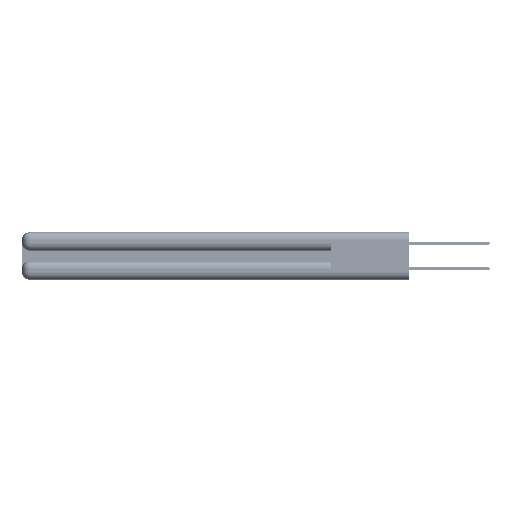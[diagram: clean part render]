
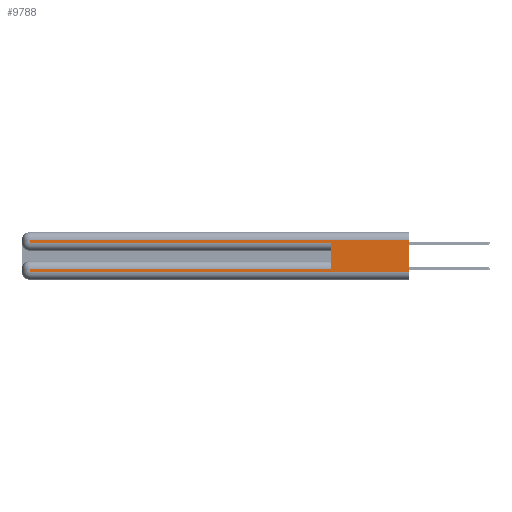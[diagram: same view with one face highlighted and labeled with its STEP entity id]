
A CAD part, left-side view. The second image highlights one B-rep face of the part: STEP entity #9788.
In plain terms, the highlighted planar face has unit normal (-1, 0, 0).
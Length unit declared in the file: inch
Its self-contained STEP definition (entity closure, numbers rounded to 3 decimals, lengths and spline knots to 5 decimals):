
#1102 = VECTOR ( 'NONE', #44371, 39.37008 ) ;
#1187 = CARTESIAN_POINT ( 'NONE',  ( 0., 0., 0.285 ) ) ;
#2878 = CARTESIAN_POINT ( 'NONE',  ( 0., 2.94, 0.285 ) ) ;
#3086 = CARTESIAN_POINT ( 'NONE',  ( 0., 0., 0.37 ) ) ;
#3756 = CARTESIAN_POINT ( 'NONE',  ( 0., 0., 0.06 ) ) ;
#4195 = CARTESIAN_POINT ( 'NONE',  ( 0., 2.94, 0.085 ) ) ;
#4802 = CARTESIAN_POINT ( 'NONE',  ( 0., 0., 0.37 ) ) ;
#5175 = DIRECTION ( 'NONE',  ( 0., 0., -1. ) ) ;
#5289 = EDGE_CURVE ( 'NONE', #52848, #55226, #8378, .T. ) ;
#5853 = LINE ( 'NONE', #35079, #46763 ) ;
#6275 = DIRECTION ( 'NONE',  ( 0., -1., 0. ) ) ;
#7104 = DIRECTION ( 'NONE',  ( 0., 0., -1. ) ) ;
#7128 = VECTOR ( 'NONE', #55482, 39.37008 ) ;
#8378 = LINE ( 'NONE', #32959, #16560 ) ;
#8469 = VERTEX_POINT ( 'NONE', #21962 ) ;
#8534 = ORIENTED_EDGE ( 'NONE', *, *, #32265, .T. ) ;
#9788 = ADVANCED_FACE ( 'NONE', ( #42349 ), #50697, .F. ) ;
#11920 = AXIS2_PLACEMENT_3D ( 'NONE', #3086, #24656, #7104 ) ;
#12340 = EDGE_CURVE ( 'NONE', #14907, #27294, #5853, .T. ) ;
#12883 = ORIENTED_EDGE ( 'NONE', *, *, #45761, .F. ) ;
#14907 = VERTEX_POINT ( 'NONE', #55323 ) ;
#15025 = DIRECTION ( 'NONE',  ( 0., 0., 1. ) ) ;
#16560 = VECTOR ( 'NONE', #36776, 39.37008 ) ;
#18267 = ORIENTED_EDGE ( 'NONE', *, *, #26750, .T. ) ;
#18658 = ORIENTED_EDGE ( 'NONE', *, *, #43704, .T. ) ;
#19375 = CARTESIAN_POINT ( 'NONE',  ( 0., 0., 0.31 ) ) ;
#20033 = CARTESIAN_POINT ( 'NONE',  ( 0., 0.6, 0.085 ) ) ;
#20605 = LINE ( 'NONE', #1187, #53283 ) ;
#21962 = CARTESIAN_POINT ( 'NONE',  ( 0., 0., 0.06 ) ) ;
#23634 = CARTESIAN_POINT ( 'NONE',  ( 0., 0.6, 0.145 ) ) ;
#24656 = DIRECTION ( 'NONE',  ( 1., 0., 0. ) ) ;
#26646 = ORIENTED_EDGE ( 'NONE', *, *, #48964, .F. ) ;
#26750 = EDGE_CURVE ( 'NONE', #38836, #52848, #28959, .T. ) ;
#27242 = CARTESIAN_POINT ( 'NONE',  ( 0., 0., 0.31 ) ) ;
#27294 = VERTEX_POINT ( 'NONE', #2878 ) ;
#28958 = VECTOR ( 'NONE', #5175, 39.37008 ) ;
#28959 = LINE ( 'NONE', #33825, #7128 ) ;
#29506 = DIRECTION ( 'NONE',  ( 0., -1., 0. ) ) ;
#29976 = VECTOR ( 'NONE', #15025, 39.37008 ) ;
#30628 = LINE ( 'NONE', #23634, #29976 ) ;
#32265 = EDGE_CURVE ( 'NONE', #34788, #14907, #47413, .T. ) ;
#32959 = CARTESIAN_POINT ( 'NONE',  ( 0., 2.94, 0.37 ) ) ;
#33825 = CARTESIAN_POINT ( 'NONE',  ( 0., 0., 0.085 ) ) ;
#34003 = CARTESIAN_POINT ( 'NONE',  ( 0., 2.94, 0.06 ) ) ;
#34576 = DIRECTION ( 'NONE',  ( 0., 0., -1. ) ) ;
#34788 = VERTEX_POINT ( 'NONE', #19375 ) ;
#35011 = ORIENTED_EDGE ( 'NONE', *, *, #12340, .T. ) ;
#35079 = CARTESIAN_POINT ( 'NONE',  ( 0., 2.94, 0.37 ) ) ;
#36162 = VECTOR ( 'NONE', #29506, 39.37008 ) ;
#36776 = DIRECTION ( 'NONE',  ( 0., 0., -1. ) ) ;
#38639 = CARTESIAN_POINT ( 'NONE',  ( 0., 0.6, 0.285 ) ) ;
#38836 = VERTEX_POINT ( 'NONE', #20033 ) ;
#40536 = LINE ( 'NONE', #4802, #28958 ) ;
#42349 = FACE_OUTER_BOUND ( 'NONE', #53322, .T. ) ;
#42494 = VERTEX_POINT ( 'NONE', #38639 ) ;
#43704 = EDGE_CURVE ( 'NONE', #27294, #42494, #20605, .T. ) ;
#44330 = ORIENTED_EDGE ( 'NONE', *, *, #5289, .T. ) ;
#44371 = DIRECTION ( 'NONE',  ( 0., 1., 0. ) ) ;
#45761 = EDGE_CURVE ( 'NONE', #38836, #42494, #30628, .T. ) ;
#46359 = LINE ( 'NONE', #3756, #36162 ) ;
#46763 = VECTOR ( 'NONE', #34576, 39.37008 ) ;
#47037 = ORIENTED_EDGE ( 'NONE', *, *, #56022, .T. ) ;
#47413 = LINE ( 'NONE', #27242, #1102 ) ;
#48964 = EDGE_CURVE ( 'NONE', #34788, #8469, #40536, .T. ) ;
#50697 = PLANE ( 'NONE',  #11920 ) ;
#52848 = VERTEX_POINT ( 'NONE', #4195 ) ;
#53283 = VECTOR ( 'NONE', #6275, 39.37008 ) ;
#53322 = EDGE_LOOP ( 'NONE', ( #26646, #8534, #35011, #18658, #12883, #18267, #44330, #47037 ) ) ;
#55226 = VERTEX_POINT ( 'NONE', #34003 ) ;
#55323 = CARTESIAN_POINT ( 'NONE',  ( 0., 2.94, 0.31 ) ) ;
#55482 = DIRECTION ( 'NONE',  ( 0., 1., 0. ) ) ;
#56022 = EDGE_CURVE ( 'NONE', #55226, #8469, #46359, .T. ) ;
